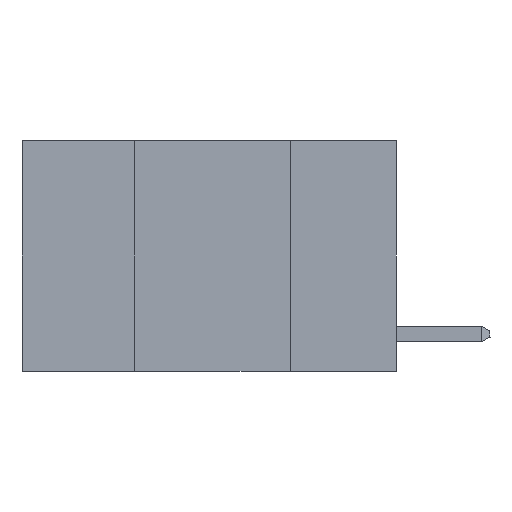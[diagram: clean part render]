
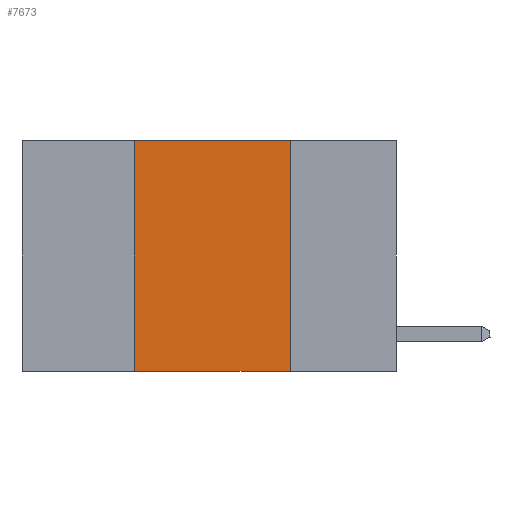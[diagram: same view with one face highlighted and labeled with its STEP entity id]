
A CAD part, left-side view. The second image highlights one B-rep face of the part: STEP entity #7673.
In plain terms, the highlighted planar face has unit normal (-1, 0, 0).
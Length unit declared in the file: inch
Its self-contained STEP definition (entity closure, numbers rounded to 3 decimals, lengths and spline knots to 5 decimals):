
#402 = CARTESIAN_POINT ( 'NONE',  ( 0., 0.17, 0. ) ) ;
#1466 = LINE ( 'NONE', #7170, #12933 ) ;
#1763 = EDGE_CURVE ( 'NONE', #11231, #12937, #12647, .T. ) ;
#1967 = LINE ( 'NONE', #402, #13759 ) ;
#2903 = FACE_OUTER_BOUND ( 'NONE', #6327, .T. ) ;
#2962 = LINE ( 'NONE', #12904, #5674 ) ;
#3552 = DIRECTION ( 'NONE',  ( 0., -1., 0. ) ) ;
#3808 = EDGE_CURVE ( 'NONE', #10506, #10681, #1466, .T. ) ;
#4104 = DIRECTION ( 'NONE',  ( 0., 0., 1. ) ) ;
#4368 = ORIENTED_EDGE ( 'NONE', *, *, #3808, .F. ) ;
#4527 = ORIENTED_EDGE ( 'NONE', *, *, #8840, .F. ) ;
#4732 = DIRECTION ( 'NONE',  ( 1., 0., 0. ) ) ;
#5476 = CARTESIAN_POINT ( 'NONE',  ( 0., 0.17, 0. ) ) ;
#5674 = VECTOR ( 'NONE', #4104, 39.37008 ) ;
#5793 = ORIENTED_EDGE ( 'NONE', *, *, #1763, .T. ) ;
#6222 = ORIENTED_EDGE ( 'NONE', *, *, #12505, .F. ) ;
#6327 = EDGE_LOOP ( 'NONE', ( #4527, #4368, #6222, #5793 ) ) ;
#7170 = CARTESIAN_POINT ( 'NONE',  ( 0., 0.6, 0. ) ) ;
#7673 = ADVANCED_FACE ( 'NONE', ( #2903 ), #13452, .F. ) ;
#8238 = DIRECTION ( 'NONE',  ( 0., 0., -1. ) ) ;
#8654 = AXIS2_PLACEMENT_3D ( 'NONE', #11361, #4732, #12427 ) ;
#8840 = EDGE_CURVE ( 'NONE', #10681, #12937, #1967, .T. ) ;
#9650 = CARTESIAN_POINT ( 'NONE',  ( 0., 0.42, -0.37 ) ) ;
#10116 = CARTESIAN_POINT ( 'NONE',  ( 0., 0.42, 0. ) ) ;
#10213 = CARTESIAN_POINT ( 'NONE',  ( 0., 0.6, -0.37 ) ) ;
#10506 = VERTEX_POINT ( 'NONE', #10116 ) ;
#10681 = VERTEX_POINT ( 'NONE', #5476 ) ;
#11231 = VERTEX_POINT ( 'NONE', #9650 ) ;
#11361 = CARTESIAN_POINT ( 'NONE',  ( 0., 0.6, 0. ) ) ;
#12427 = DIRECTION ( 'NONE',  ( 0., 0., -1. ) ) ;
#12505 = EDGE_CURVE ( 'NONE', #11231, #10506, #2962, .T. ) ;
#12647 = LINE ( 'NONE', #10213, #13642 ) ;
#12766 = CARTESIAN_POINT ( 'NONE',  ( 0., 0.17, -0.37 ) ) ;
#12904 = CARTESIAN_POINT ( 'NONE',  ( 0., 0.42, 0. ) ) ;
#12933 = VECTOR ( 'NONE', #13657, 39.37008 ) ;
#12937 = VERTEX_POINT ( 'NONE', #12766 ) ;
#13452 = PLANE ( 'NONE',  #8654 ) ;
#13642 = VECTOR ( 'NONE', #3552, 39.37008 ) ;
#13657 = DIRECTION ( 'NONE',  ( 0., -1., 0. ) ) ;
#13759 = VECTOR ( 'NONE', #8238, 39.37008 ) ;
